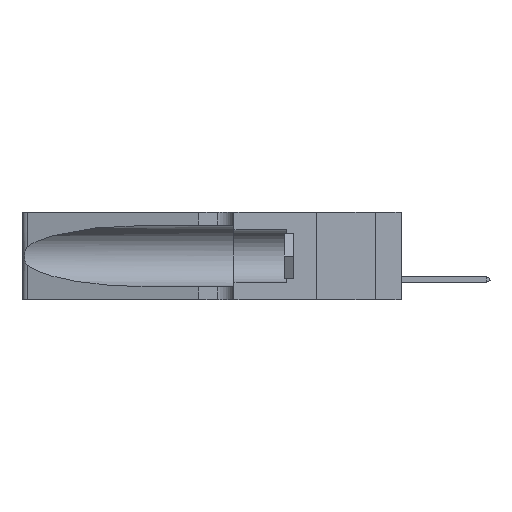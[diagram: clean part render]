
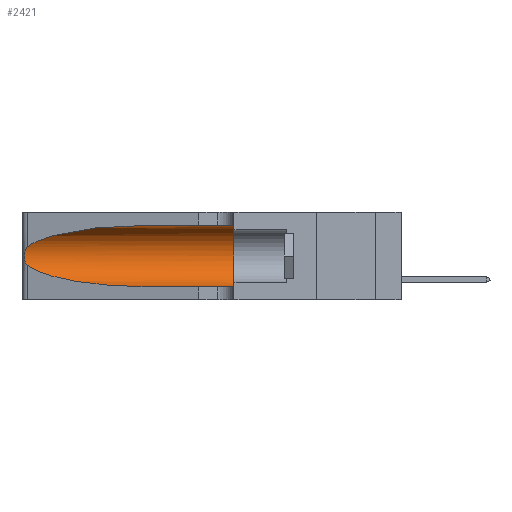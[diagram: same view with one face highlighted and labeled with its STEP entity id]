
A CAD part, left-side view. The second image highlights one B-rep face of the part: STEP entity #2421.
In plain terms, the highlighted cylindrical face has radius 3.308 mm (diameter 6.617 mm), a partial arc.
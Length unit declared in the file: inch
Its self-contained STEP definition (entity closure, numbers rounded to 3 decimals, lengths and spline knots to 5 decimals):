
#2396 = CARTESIAN_POINT ( 'NONE',  ( 0.1305, 0.35, 0.31525 ) ) ;
#2421 = ADVANCED_FACE ( 'NONE', ( #29164 ), #11174, .F. ) ;
#3167 = CARTESIAN_POINT ( 'NONE',  ( 0.25555, 1.22994, 0.2215 ) ) ;
#3291 = CARTESIAN_POINT ( 'NONE',  ( 0.25487, 1.22718, 0.22369 ) ) ;
#3417 = CARTESIAN_POINT ( 'NONE',  ( 0.26017, 1.23833, 0.17102 ) ) ;
#4039 = LINE ( 'NONE', #27945, #23240 ) ;
#4174 = VERTEX_POINT ( 'NONE', #23372 ) ;
#4283 =( BOUNDED_CURVE ( )  B_SPLINE_CURVE ( 3, ( #15415, #33791, #26145, #23216 ),
 .UNSPECIFIED., .F., .F. ) 
 B_SPLINE_CURVE_WITH_KNOTS ( ( 4, 4 ),
 ( 1.5708, 2.84003 ),
 .UNSPECIFIED. ) 
 CURVE ( )  GEOMETRIC_REPRESENTATION_ITEM ( )  RATIONAL_B_SPLINE_CURVE ( ( 1., 0.87, 0.87, 1. ) ) 
 REPRESENTATION_ITEM ( '' )  );
#4495 = VERTEX_POINT ( 'NONE', #24966 ) ;
#5142 = DIRECTION ( 'NONE',  ( 0., 0., 1. ) ) ;
#5735 = CARTESIAN_POINT ( 'NONE',  ( 0.2373, 1.15595, 0.08982 ) ) ;
#5978 = CARTESIAN_POINT ( 'NONE',  ( 0.25555, 1.22993, 0.14849 ) ) ;
#6197 = CARTESIAN_POINT ( 'NONE',  ( 0.25787, 1.23484, 0.2124 ) ) ;
#6703 = ORIENTED_EDGE ( 'NONE', *, *, #29490, .F. ) ;
#7740 = ORIENTED_EDGE ( 'NONE', *, *, #29933, .T. ) ;
#8314 =( BOUNDED_CURVE ( )  B_SPLINE_CURVE ( 3, ( #21728, #5735, #21517, #10890 ),
 .UNSPECIFIED., .F., .T. ) 
 B_SPLINE_CURVE_WITH_KNOTS ( ( 4, 4 ),
 ( 3.44316, 4.71239 ),
 .UNSPECIFIED. ) 
 CURVE ( )  GEOMETRIC_REPRESENTATION_ITEM ( )  RATIONAL_B_SPLINE_CURVE ( ( 1., 0.87, 0.87, 1. ) ) 
 REPRESENTATION_ITEM ( '' )  );
#8316 = AXIS2_PLACEMENT_3D ( 'NONE', #9825, #23949, #5142 ) ;
#8526 = CARTESIAN_POINT ( 'NONE',  ( 0.26018, 1.23835, 0.19895 ) ) ;
#8583 = CARTESIAN_POINT ( 'NONE',  ( 0.1305, 0.72297, 0.05475 ) ) ;
#9825 = CARTESIAN_POINT ( 'NONE',  ( 0.1305, 0.35, 0.185 ) ) ;
#10457 = CARTESIAN_POINT ( 'NONE',  ( 0.25487, 1.22718, 0.14631 ) ) ;
#10890 = CARTESIAN_POINT ( 'NONE',  ( 0.1305, 0.72297, 0.05475 ) ) ;
#11174 = CYLINDRICAL_SURFACE ( 'NONE', #27142, 0.13025 ) ;
#12117 = EDGE_CURVE ( 'NONE', #21513, #18888, #21628, .T. ) ;
#12415 = ORIENTED_EDGE ( 'NONE', *, *, #14778, .T. ) ;
#14302 = EDGE_CURVE ( 'NONE', #4174, #25754, #26946, .T. ) ;
#14778 = EDGE_CURVE ( 'NONE', #17951, #18888, #22774, .T. ) ;
#15415 = CARTESIAN_POINT ( 'NONE',  ( 0.1305, 0.72297, 0.31525 ) ) ;
#16253 = ORIENTED_EDGE ( 'NONE', *, *, #14302, .T. ) ;
#16487 = CARTESIAN_POINT ( 'NONE',  ( 0.25856, 1.23593, 0.16098 ) ) ;
#16604 = CARTESIAN_POINT ( 'NONE',  ( 0.25639, 1.23186, 0.15144 ) ) ;
#17951 = VERTEX_POINT ( 'NONE', #8583 ) ;
#18614 = DIRECTION ( 'NONE',  ( 0., -1., 0. ) ) ;
#18888 = VERTEX_POINT ( 'NONE', #24612 ) ;
#20568 = ORIENTED_EDGE ( 'NONE', *, *, #12117, .F. ) ;
#21476 = DIRECTION ( 'NONE',  ( 0., 0., -1. ) ) ;
#21513 = VERTEX_POINT ( 'NONE', #2396 ) ;
#21517 = CARTESIAN_POINT ( 'NONE',  ( 0.18966, 0.96281, 0.05475 ) ) ;
#21628 = CIRCLE ( 'NONE', #8316, 0.13025 ) ;
#21728 = CARTESIAN_POINT ( 'NONE',  ( 0.25487, 1.22718, 0.14631 ) ) ;
#21803 = CARTESIAN_POINT ( 'NONE',  ( 0.1305, 1.61858, 0.185 ) ) ;
#22201 = CARTESIAN_POINT ( 'NONE',  ( 0.25854, 1.2359, 0.20912 ) ) ;
#22774 = LINE ( 'NONE', #31887, #24016 ) ;
#23216 = CARTESIAN_POINT ( 'NONE',  ( 0.25487, 1.22718, 0.22369 ) ) ;
#23240 = VECTOR ( 'NONE', #26658, 39.37008 ) ;
#23372 = CARTESIAN_POINT ( 'NONE',  ( 0.25487, 1.22718, 0.22369 ) ) ;
#23949 = DIRECTION ( 'NONE',  ( 0., 1., 0. ) ) ;
#24016 = VECTOR ( 'NONE', #18614, 39.37008 ) ;
#24490 = DIRECTION ( 'NONE',  ( 0., -1., 0. ) ) ;
#24612 = CARTESIAN_POINT ( 'NONE',  ( 0.1305, 0.35, 0.05475 ) ) ;
#24966 = CARTESIAN_POINT ( 'NONE',  ( 0.1305, 0.72297, 0.31525 ) ) ;
#25200 = ORIENTED_EDGE ( 'NONE', *, *, #28093, .T. ) ;
#25754 = VERTEX_POINT ( 'NONE', #10457 ) ;
#26145 = CARTESIAN_POINT ( 'NONE',  ( 0.2373, 1.15595, 0.28018 ) ) ;
#26658 = DIRECTION ( 'NONE',  ( 0., -1., 0. ) ) ;
#26946 = B_SPLINE_CURVE_WITH_KNOTS ( 'NONE', 3,
 ( #3291, #3167, #32891, #6197, #22201, #8526, #32681, #32554, #3417, #16487, #32789, #16604, #5978, #27216 ),
 .UNSPECIFIED., .F., .F.,
 ( 4, 2, 2, 2, 2, 2, 4 ),
 ( 0., 0.00027, 0.00053, 0.00107, 0.0016, 0.00187, 0.00214 ),
 .UNSPECIFIED. ) ;
#27142 = AXIS2_PLACEMENT_3D ( 'NONE', #21803, #24490, #21476 ) ;
#27216 = CARTESIAN_POINT ( 'NONE',  ( 0.25487, 1.22718, 0.14631 ) ) ;
#27945 = CARTESIAN_POINT ( 'NONE',  ( 0.1305, 1.61858, 0.31525 ) ) ;
#28093 = EDGE_CURVE ( 'NONE', #25754, #17951, #8314, .T. ) ;
#29164 = FACE_OUTER_BOUND ( 'NONE', #29474, .T. ) ;
#29474 = EDGE_LOOP ( 'NONE', ( #7740, #16253, #25200, #12415, #20568, #6703 ) ) ;
#29490 = EDGE_CURVE ( 'NONE', #4495, #21513, #4039, .T. ) ;
#29933 = EDGE_CURVE ( 'NONE', #4495, #4174, #4283, .T. ) ;
#31887 = CARTESIAN_POINT ( 'NONE',  ( 0.1305, 1.61858, 0.05475 ) ) ;
#32554 = CARTESIAN_POINT ( 'NONE',  ( 0.26075, 1.23896, 0.178 ) ) ;
#32681 = CARTESIAN_POINT ( 'NONE',  ( 0.26075, 1.23896, 0.19203 ) ) ;
#32789 = CARTESIAN_POINT ( 'NONE',  ( 0.25789, 1.23486, 0.15765 ) ) ;
#32891 = CARTESIAN_POINT ( 'NONE',  ( 0.25639, 1.23184, 0.21858 ) ) ;
#33791 = CARTESIAN_POINT ( 'NONE',  ( 0.18966, 0.96281, 0.31525 ) ) ;
